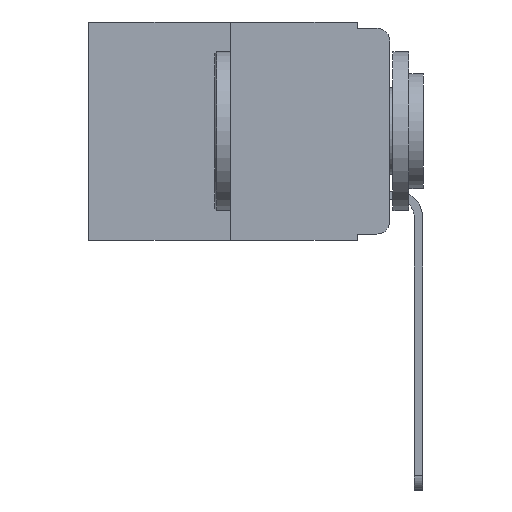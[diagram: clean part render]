
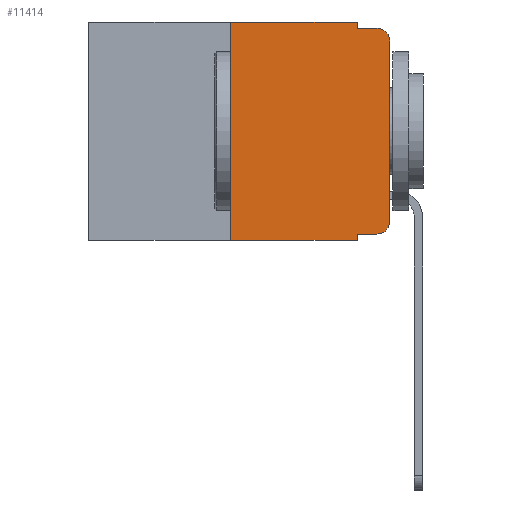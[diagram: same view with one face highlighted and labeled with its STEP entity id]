
A CAD part, left-side view. The second image highlights one B-rep face of the part: STEP entity #11414.
In plain terms, the highlighted planar face has unit normal (-1, 0, 0).
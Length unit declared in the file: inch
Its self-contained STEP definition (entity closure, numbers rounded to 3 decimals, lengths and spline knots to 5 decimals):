
#52 = DIRECTION ( 'NONE',  ( 0., 0., -1. ) ) ;
#235 = VERTEX_POINT ( 'NONE', #13204 ) ;
#262 = ORIENTED_EDGE ( 'NONE', *, *, #5251, .T. ) ;
#356 = EDGE_CURVE ( 'NONE', #12279, #2646, #730, .T. ) ;
#357 = VECTOR ( 'NONE', #12758, 39.37008 ) ;
#461 = CARTESIAN_POINT ( 'NONE',  ( 0., 0.473, 0. ) ) ;
#526 = CARTESIAN_POINT ( 'NONE',  ( 0., 0., 0. ) ) ;
#542 = DIRECTION ( 'NONE',  ( 0., 0., -1. ) ) ;
#697 = DIRECTION ( 'NONE',  ( 0., 0., -1. ) ) ;
#730 = LINE ( 'NONE', #13214, #357 ) ;
#816 = ORIENTED_EDGE ( 'NONE', *, *, #1705, .F. ) ;
#907 = LINE ( 'NONE', #10101, #9291 ) ;
#950 = DIRECTION ( 'NONE',  ( 0., 0., -1. ) ) ;
#1177 = EDGE_CURVE ( 'NONE', #10024, #1613, #9428, .T. ) ;
#1195 = ORIENTED_EDGE ( 'NONE', *, *, #356, .F. ) ;
#1354 = VERTEX_POINT ( 'NONE', #9592 ) ;
#1613 = VERTEX_POINT ( 'NONE', #7647 ) ;
#1705 = EDGE_CURVE ( 'NONE', #2646, #1354, #1832, .T. ) ;
#1832 = LINE ( 'NONE', #8324, #7733 ) ;
#2423 = DIRECTION ( 'NONE',  ( 0., -1., 0. ) ) ;
#2572 = VECTOR ( 'NONE', #3939, 39.37008 ) ;
#2646 = VERTEX_POINT ( 'NONE', #9582 ) ;
#2942 = DIRECTION ( 'NONE',  ( 0., 0., 1. ) ) ;
#3911 = EDGE_CURVE ( 'NONE', #1354, #235, #9680, .T. ) ;
#3939 = DIRECTION ( 'NONE',  ( 0., 0., 1. ) ) ;
#4200 = CARTESIAN_POINT ( 'NONE',  ( 0., 0., -0.313 ) ) ;
#4469 = ORIENTED_EDGE ( 'NONE', *, *, #12943, .F. ) ;
#4904 = EDGE_CURVE ( 'NONE', #9625, #1613, #7894, .T. ) ;
#4966 = DIRECTION ( 'NONE',  ( 1., 0., 0. ) ) ;
#5158 = ORIENTED_EDGE ( 'NONE', *, *, #4904, .F. ) ;
#5195 = AXIS2_PLACEMENT_3D ( 'NONE', #461, #4966, #11976 ) ;
#5251 = EDGE_CURVE ( 'NONE', #10027, #12317, #11467, .T. ) ;
#5348 = EDGE_CURVE ( 'NONE', #8061, #235, #7561, .T. ) ;
#5406 = FACE_OUTER_BOUND ( 'NONE', #12474, .T. ) ;
#5494 = CARTESIAN_POINT ( 'NONE',  ( 0., 0.051, -0.333 ) ) ;
#5609 = CARTESIAN_POINT ( 'NONE',  ( 0., 0.051, 0. ) ) ;
#6365 = VECTOR ( 'NONE', #7834, 39.37008 ) ;
#7061 = DIRECTION ( 'NONE',  ( -1., 0., 0. ) ) ;
#7187 = DIRECTION ( 'NONE',  ( -1., 0., 0. ) ) ;
#7561 = CIRCLE ( 'NONE', #11867, 0.02 ) ;
#7647 = CARTESIAN_POINT ( 'NONE',  ( 0., 0.051, -0.343 ) ) ;
#7733 = VECTOR ( 'NONE', #950, 39.37008 ) ;
#7834 = DIRECTION ( 'NONE',  ( 0., -1., 0. ) ) ;
#7894 = LINE ( 'NONE', #5609, #13148 ) ;
#8061 = VERTEX_POINT ( 'NONE', #8315 ) ;
#8149 = ORIENTED_EDGE ( 'NONE', *, *, #11297, .T. ) ;
#8190 = DIRECTION ( 'NONE',  ( 0., -1., 0. ) ) ;
#8305 = ORIENTED_EDGE ( 'NONE', *, *, #10726, .T. ) ;
#8315 = CARTESIAN_POINT ( 'NONE',  ( 0., 0., -0.03 ) ) ;
#8324 = CARTESIAN_POINT ( 'NONE',  ( 0., 0.051, 0. ) ) ;
#8596 = CARTESIAN_POINT ( 'NONE',  ( 0., 0.051, -0.01 ) ) ;
#8601 = ORIENTED_EDGE ( 'NONE', *, *, #5348, .T. ) ;
#8999 = CARTESIAN_POINT ( 'NONE',  ( 0., 0.25, -0.343 ) ) ;
#9291 = VECTOR ( 'NONE', #2942, 39.37008 ) ;
#9428 = LINE ( 'NONE', #10451, #11781 ) ;
#9582 = CARTESIAN_POINT ( 'NONE',  ( 0., 0.051, 0. ) ) ;
#9592 = CARTESIAN_POINT ( 'NONE',  ( 0., 0.051, -0.01 ) ) ;
#9625 = VERTEX_POINT ( 'NONE', #5494 ) ;
#9680 = LINE ( 'NONE', #8596, #12033 ) ;
#9835 = CARTESIAN_POINT ( 'NONE',  ( 0., 0.051, -0.333 ) ) ;
#10024 = VERTEX_POINT ( 'NONE', #8999 ) ;
#10027 = VERTEX_POINT ( 'NONE', #13019 ) ;
#10101 = CARTESIAN_POINT ( 'NONE',  ( 0., 0.25, 0. ) ) ;
#10451 = CARTESIAN_POINT ( 'NONE',  ( 0., 0.473, -0.343 ) ) ;
#10552 = AXIS2_PLACEMENT_3D ( 'NONE', #12979, #7061, #542 ) ;
#10726 = EDGE_CURVE ( 'NONE', #12317, #8061, #10756, .T. ) ;
#10756 = LINE ( 'NONE', #526, #2572 ) ;
#10992 = PLANE ( 'NONE',  #5195 ) ;
#11171 = CARTESIAN_POINT ( 'NONE',  ( 0., 0.25, 0. ) ) ;
#11297 = EDGE_CURVE ( 'NONE', #9625, #10027, #12285, .T. ) ;
#11414 = ADVANCED_FACE ( 'NONE', ( #5406 ), #10992, .F. ) ;
#11467 = CIRCLE ( 'NONE', #10552, 0.02 ) ;
#11572 = ORIENTED_EDGE ( 'NONE', *, *, #3911, .F. ) ;
#11781 = VECTOR ( 'NONE', #8190, 39.37008 ) ;
#11867 = AXIS2_PLACEMENT_3D ( 'NONE', #13091, #7187, #697 ) ;
#11976 = DIRECTION ( 'NONE',  ( 0., 0., -1. ) ) ;
#12033 = VECTOR ( 'NONE', #2423, 39.37008 ) ;
#12279 = VERTEX_POINT ( 'NONE', #11171 ) ;
#12285 = LINE ( 'NONE', #9835, #6365 ) ;
#12317 = VERTEX_POINT ( 'NONE', #4200 ) ;
#12474 = EDGE_LOOP ( 'NONE', ( #8305, #8601, #11572, #816, #1195, #4469, #12810, #5158, #8149, #262 ) ) ;
#12758 = DIRECTION ( 'NONE',  ( 0., -1., 0. ) ) ;
#12810 = ORIENTED_EDGE ( 'NONE', *, *, #1177, .T. ) ;
#12943 = EDGE_CURVE ( 'NONE', #10024, #12279, #907, .T. ) ;
#12979 = CARTESIAN_POINT ( 'NONE',  ( 0., 0.02, -0.313 ) ) ;
#13019 = CARTESIAN_POINT ( 'NONE',  ( 0., 0.02, -0.333 ) ) ;
#13091 = CARTESIAN_POINT ( 'NONE',  ( 0., 0.02, -0.03 ) ) ;
#13148 = VECTOR ( 'NONE', #52, 39.37008 ) ;
#13204 = CARTESIAN_POINT ( 'NONE',  ( 0., 0.02, -0.01 ) ) ;
#13214 = CARTESIAN_POINT ( 'NONE',  ( 0., 0.473, 0. ) ) ;
